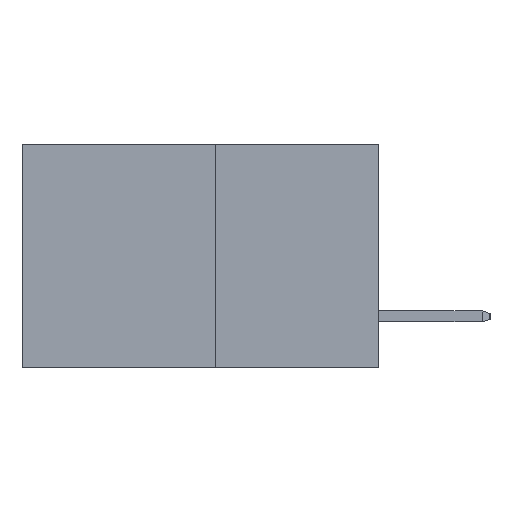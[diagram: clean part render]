
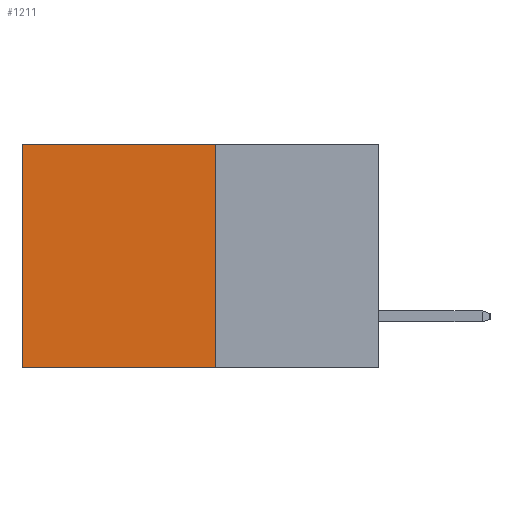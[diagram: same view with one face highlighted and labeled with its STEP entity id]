
A CAD part, left-side view. The second image highlights one B-rep face of the part: STEP entity #1211.
In plain terms, the highlighted planar face has unit normal (-1, 0, 0).
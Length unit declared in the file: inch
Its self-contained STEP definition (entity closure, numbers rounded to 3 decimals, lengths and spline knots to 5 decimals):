
#496 = VERTEX_POINT ( 'NONE', #12225 ) ;
#1211 = ADVANCED_FACE ( 'NONE', ( #7964 ), #1724, .F. ) ;
#1601 = CARTESIAN_POINT ( 'NONE',  ( 0.277, 0.27, -0.37 ) ) ;
#1664 = DIRECTION ( 'NONE',  ( 1., 0., 0. ) ) ;
#1697 = DIRECTION ( 'NONE',  ( 0., 1., 0. ) ) ;
#1724 = PLANE ( 'NONE',  #13097 ) ;
#2344 = VECTOR ( 'NONE', #8636, 39.37008 ) ;
#3175 = CARTESIAN_POINT ( 'NONE',  ( 0.277, 0.59, -0.37 ) ) ;
#3635 = CARTESIAN_POINT ( 'NONE',  ( 0.277, 0.27, -0.37 ) ) ;
#4420 = VERTEX_POINT ( 'NONE', #4598 ) ;
#4598 = CARTESIAN_POINT ( 'NONE',  ( 0.277, 0.59, 0. ) ) ;
#4760 = VECTOR ( 'NONE', #11779, 39.37008 ) ;
#5240 = VERTEX_POINT ( 'NONE', #9814 ) ;
#6507 = VECTOR ( 'NONE', #6520, 39.37008 ) ;
#6520 = DIRECTION ( 'NONE',  ( 0., 0., -1. ) ) ;
#7719 = LINE ( 'NONE', #10741, #4760 ) ;
#7964 = FACE_OUTER_BOUND ( 'NONE', #13470, .T. ) ;
#8225 = LINE ( 'NONE', #10512, #13443 ) ;
#8636 = DIRECTION ( 'NONE',  ( 0., 0., -1. ) ) ;
#8655 = VERTEX_POINT ( 'NONE', #3635 ) ;
#9412 = LINE ( 'NONE', #3175, #6507 ) ;
#9814 = CARTESIAN_POINT ( 'NONE',  ( 0.277, 0.59, -0.37 ) ) ;
#10512 = CARTESIAN_POINT ( 'NONE',  ( 0.277, 0.27, 0. ) ) ;
#10741 = CARTESIAN_POINT ( 'NONE',  ( 0.277, 0.27, -0.37 ) ) ;
#11055 = DIRECTION ( 'NONE',  ( 0., 0., -1. ) ) ;
#11330 = EDGE_CURVE ( 'NONE', #4420, #5240, #9412, .T. ) ;
#11512 = ORIENTED_EDGE ( 'NONE', *, *, #11330, .T. ) ;
#11779 = DIRECTION ( 'NONE',  ( 0., 1., 0. ) ) ;
#11900 = EDGE_CURVE ( 'NONE', #8655, #5240, #7719, .T. ) ;
#12225 = CARTESIAN_POINT ( 'NONE',  ( 0.277, 0.27, 0. ) ) ;
#12452 = ORIENTED_EDGE ( 'NONE', *, *, #12705, .F. ) ;
#12705 = EDGE_CURVE ( 'NONE', #496, #8655, #13771, .T. ) ;
#13084 = ORIENTED_EDGE ( 'NONE', *, *, #11900, .F. ) ;
#13097 = AXIS2_PLACEMENT_3D ( 'NONE', #1601, #1664, #11055 ) ;
#13242 = ORIENTED_EDGE ( 'NONE', *, *, #13957, .T. ) ;
#13443 = VECTOR ( 'NONE', #1697, 39.37008 ) ;
#13470 = EDGE_LOOP ( 'NONE', ( #11512, #13084, #12452, #13242 ) ) ;
#13771 = LINE ( 'NONE', #13783, #2344 ) ;
#13783 = CARTESIAN_POINT ( 'NONE',  ( 0.277, 0.27, -0.37 ) ) ;
#13957 = EDGE_CURVE ( 'NONE', #496, #4420, #8225, .T. ) ;
